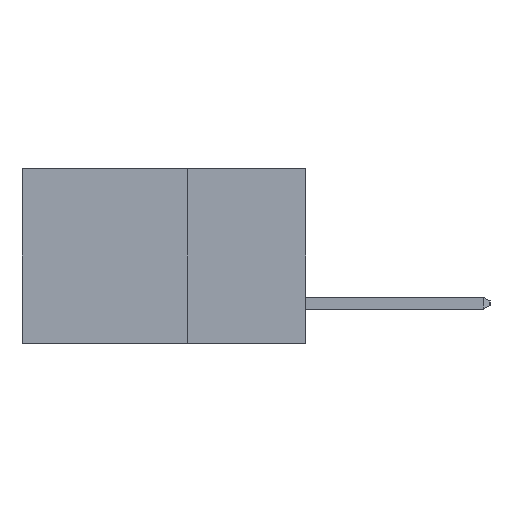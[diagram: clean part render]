
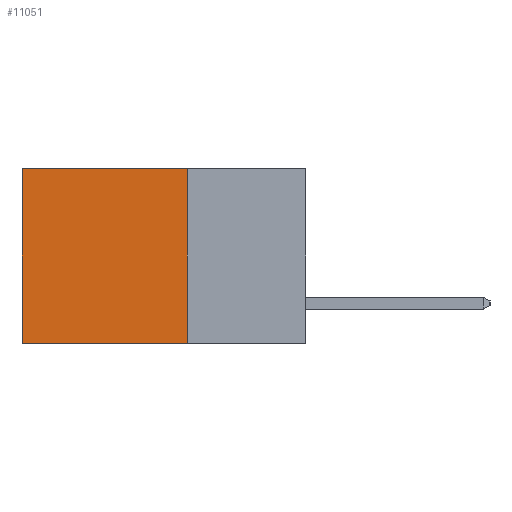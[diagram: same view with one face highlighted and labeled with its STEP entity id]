
A CAD part, left-side view. The second image highlights one B-rep face of the part: STEP entity #11051.
In plain terms, the highlighted planar face has unit normal (-1, 0, 0).
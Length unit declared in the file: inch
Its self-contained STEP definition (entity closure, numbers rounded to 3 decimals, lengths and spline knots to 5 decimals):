
#918 = ORIENTED_EDGE ( 'NONE', *, *, #32131, .F. ) ;
#1863 = DIRECTION ( 'NONE',  ( 0., 1., 0. ) ) ;
#2484 = VECTOR ( 'NONE', #5562, 39.37008 ) ;
#3846 = VECTOR ( 'NONE', #1863, 39.37008 ) ;
#5130 = CARTESIAN_POINT ( 'NONE',  ( 0.298, 0.25, -0.37 ) ) ;
#5562 = DIRECTION ( 'NONE',  ( 0., 1., 0. ) ) ;
#5663 = CARTESIAN_POINT ( 'NONE',  ( 0.298, 0.25, -0.37 ) ) ;
#6968 = LINE ( 'NONE', #26674, #19834 ) ;
#7575 = CARTESIAN_POINT ( 'NONE',  ( 0.298, 0.6, 0. ) ) ;
#9105 = EDGE_CURVE ( 'NONE', #28949, #14353, #24908, .T. ) ;
#9231 = PLANE ( 'NONE',  #23431 ) ;
#10593 = LINE ( 'NONE', #19672, #3846 ) ;
#11051 = ADVANCED_FACE ( 'NONE', ( #27799 ), #9231, .F. ) ;
#11773 = DIRECTION ( 'NONE',  ( 1., 0., 0. ) ) ;
#11980 = VECTOR ( 'NONE', #22980, 39.37008 ) ;
#12210 = ORIENTED_EDGE ( 'NONE', *, *, #15376, .T. ) ;
#13710 = VERTEX_POINT ( 'NONE', #5130 ) ;
#13900 = DIRECTION ( 'NONE',  ( 0., 0., -1. ) ) ;
#14353 = VERTEX_POINT ( 'NONE', #17919 ) ;
#15376 = EDGE_CURVE ( 'NONE', #17626, #28949, #10593, .T. ) ;
#17626 = VERTEX_POINT ( 'NONE', #23226 ) ;
#17919 = CARTESIAN_POINT ( 'NONE',  ( 0.298, 0.6, -0.37 ) ) ;
#19672 = CARTESIAN_POINT ( 'NONE',  ( 0.298, 0.25, 0. ) ) ;
#19834 = VECTOR ( 'NONE', #13900, 39.37008 ) ;
#22179 = CARTESIAN_POINT ( 'NONE',  ( 0.298, 0.6, 0. ) ) ;
#22980 = DIRECTION ( 'NONE',  ( 0., 0., -1. ) ) ;
#23226 = CARTESIAN_POINT ( 'NONE',  ( 0.298, 0.25, 0. ) ) ;
#23431 = AXIS2_PLACEMENT_3D ( 'NONE', #27145, #11773, #29732 ) ;
#24908 = LINE ( 'NONE', #7575, #11980 ) ;
#25105 = ORIENTED_EDGE ( 'NONE', *, *, #9105, .T. ) ;
#26195 = ORIENTED_EDGE ( 'NONE', *, *, #27687, .F. ) ;
#26674 = CARTESIAN_POINT ( 'NONE',  ( 0.298, 0.25, 0. ) ) ;
#27145 = CARTESIAN_POINT ( 'NONE',  ( 0.298, 0.25, 0. ) ) ;
#27687 = EDGE_CURVE ( 'NONE', #13710, #14353, #28073, .T. ) ;
#27799 = FACE_OUTER_BOUND ( 'NONE', #28918, .T. ) ;
#28073 = LINE ( 'NONE', #5663, #2484 ) ;
#28918 = EDGE_LOOP ( 'NONE', ( #25105, #26195, #918, #12210 ) ) ;
#28949 = VERTEX_POINT ( 'NONE', #22179 ) ;
#29732 = DIRECTION ( 'NONE',  ( 0., 0., -1. ) ) ;
#32131 = EDGE_CURVE ( 'NONE', #17626, #13710, #6968, .T. ) ;
